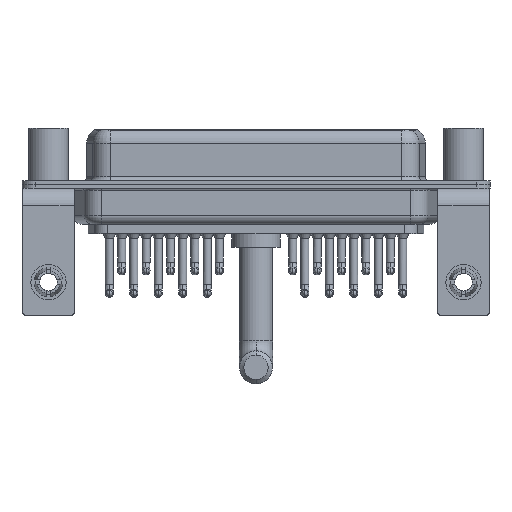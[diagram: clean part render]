
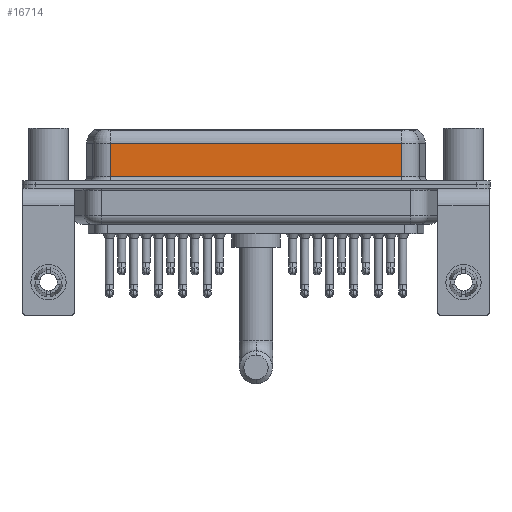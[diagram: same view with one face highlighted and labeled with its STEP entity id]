
A CAD part, front view. The second image highlights one B-rep face of the part: STEP entity #16714.
In plain terms, the highlighted planar face has unit normal (0, -1, 0).
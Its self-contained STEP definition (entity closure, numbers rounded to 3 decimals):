
#376 = DIRECTION ( 'NONE',  ( 0., 1., 0. ) ) ;
#1013 = CARTESIAN_POINT ( 'NONE',  ( 40.037, -3.95, 4.65 ) ) ;
#1127 = EDGE_CURVE ( 'NONE', #2904, #6858, #20053, .T. ) ;
#2904 = VERTEX_POINT ( 'NONE', #1013 ) ;
#4084 = LINE ( 'NONE', #10067, #17499 ) ;
#4626 = CARTESIAN_POINT ( 'NONE',  ( 7.013, -3.95, 6.4 ) ) ;
#4627 = DIRECTION ( 'NONE',  ( 0., 0., 1. ) ) ;
#5737 = CARTESIAN_POINT ( 'NONE',  ( 40.037, -3.95, 4.65 ) ) ;
#6858 = VERTEX_POINT ( 'NONE', #19440 ) ;
#7074 = ORIENTED_EDGE ( 'NONE', *, *, #18443, .F. ) ;
#8631 = DIRECTION ( 'NONE',  ( 0., 0., -1. ) ) ;
#8642 = ORIENTED_EDGE ( 'NONE', *, *, #1127, .T. ) ;
#10067 = CARTESIAN_POINT ( 'NONE',  ( 40.037, -3.95, 6.4 ) ) ;
#10706 = AXIS2_PLACEMENT_3D ( 'NONE', #16572, #376, #4627 ) ;
#10859 = LINE ( 'NONE', #4626, #12831 ) ;
#11512 = CARTESIAN_POINT ( 'NONE',  ( 40.037, -3.95, 0.9 ) ) ;
#12344 = VECTOR ( 'NONE', #13376, 1000. ) ;
#12602 = EDGE_CURVE ( 'NONE', #6858, #18048, #10859, .T. ) ;
#12831 = VECTOR ( 'NONE', #8631, 1000. ) ;
#13376 = DIRECTION ( 'NONE',  ( 1., 0., 0. ) ) ;
#15632 = LINE ( 'NONE', #11512, #12344 ) ;
#15864 = ORIENTED_EDGE ( 'NONE', *, *, #15965, .T. ) ;
#15965 = EDGE_CURVE ( 'NONE', #18048, #23704, #15632, .T. ) ;
#16572 = CARTESIAN_POINT ( 'NONE',  ( 40.037, -3.95, 6.4 ) ) ;
#16714 = ADVANCED_FACE ( 'NONE', ( #18574 ), #16960, .F. ) ;
#16834 = CARTESIAN_POINT ( 'NONE',  ( 40.037, -3.95, 0.9 ) ) ;
#16960 = PLANE ( 'NONE',  #10706 ) ;
#17499 = VECTOR ( 'NONE', #24224, 1000. ) ;
#17573 = ORIENTED_EDGE ( 'NONE', *, *, #12602, .T. ) ;
#18048 = VERTEX_POINT ( 'NONE', #18312 ) ;
#18312 = CARTESIAN_POINT ( 'NONE',  ( 7.013, -3.95, 0.9 ) ) ;
#18443 = EDGE_CURVE ( 'NONE', #2904, #23704, #4084, .T. ) ;
#18535 = VECTOR ( 'NONE', #22297, 1000. ) ;
#18574 = FACE_OUTER_BOUND ( 'NONE', #25000, .T. ) ;
#19440 = CARTESIAN_POINT ( 'NONE',  ( 7.013, -3.95, 4.65 ) ) ;
#20053 = LINE ( 'NONE', #5737, #18535 ) ;
#22297 = DIRECTION ( 'NONE',  ( -1., 0., 0. ) ) ;
#23704 = VERTEX_POINT ( 'NONE', #16834 ) ;
#24224 = DIRECTION ( 'NONE',  ( 0., 0., -1. ) ) ;
#25000 = EDGE_LOOP ( 'NONE', ( #7074, #8642, #17573, #15864 ) ) ;
